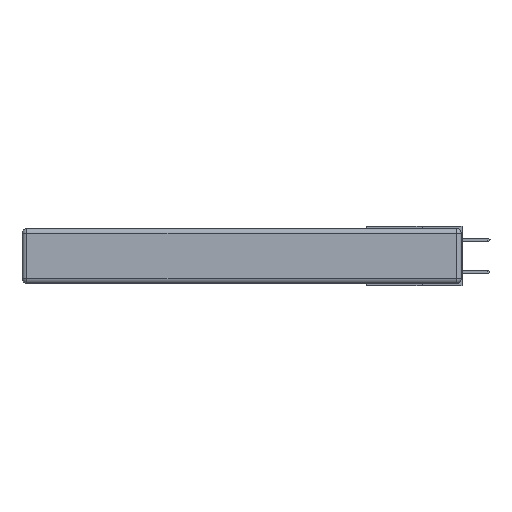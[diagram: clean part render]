
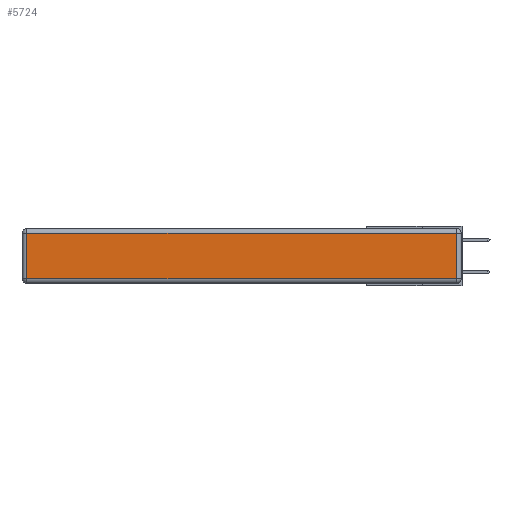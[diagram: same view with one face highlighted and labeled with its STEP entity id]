
A CAD part, left-side view. The second image highlights one B-rep face of the part: STEP entity #5724.
In plain terms, the highlighted planar face has unit normal (-1, 0, 0).
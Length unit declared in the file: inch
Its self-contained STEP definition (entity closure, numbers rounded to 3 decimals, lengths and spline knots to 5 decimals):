
#425 = CARTESIAN_POINT ( 'NONE',  ( 0., 0., -0.343 ) ) ;
#998 = CARTESIAN_POINT ( 'NONE',  ( 0., 2.72, -0.313 ) ) ;
#1907 = EDGE_CURVE ( 'NONE', #13827, #5685, #7964, .T. ) ;
#1959 = VECTOR ( 'NONE', #6742, 39.37008 ) ;
#2517 = DIRECTION ( 'NONE',  ( -1., 0., 0. ) ) ;
#2573 = DIRECTION ( 'NONE',  ( 0., 0., 1. ) ) ;
#3725 = ORIENTED_EDGE ( 'NONE', *, *, #9634, .T. ) ;
#4074 = DIRECTION ( 'NONE',  ( 0., 0., -1. ) ) ;
#4792 = VERTEX_POINT ( 'NONE', #12537 ) ;
#5685 = VERTEX_POINT ( 'NONE', #10365 ) ;
#5724 = ADVANCED_FACE ( 'NONE', ( #11742 ), #8298, .T. ) ;
#5880 = ORIENTED_EDGE ( 'NONE', *, *, #1907, .T. ) ;
#6145 = VECTOR ( 'NONE', #4074, 39.37008 ) ;
#6176 = CARTESIAN_POINT ( 'NONE',  ( 0., 2.75, -0.03 ) ) ;
#6742 = DIRECTION ( 'NONE',  ( 0., 0., 1. ) ) ;
#6750 = ORIENTED_EDGE ( 'NONE', *, *, #9700, .T. ) ;
#6792 = LINE ( 'NONE', #8973, #1959 ) ;
#6838 = DIRECTION ( 'NONE',  ( 0., -1., 0. ) ) ;
#7444 = VECTOR ( 'NONE', #6838, 39.37008 ) ;
#7964 = LINE ( 'NONE', #12325, #7444 ) ;
#8114 = VECTOR ( 'NONE', #8512, 39.37008 ) ;
#8298 = PLANE ( 'NONE',  #14353 ) ;
#8512 = DIRECTION ( 'NONE',  ( 0., 1., 0. ) ) ;
#8834 = CARTESIAN_POINT ( 'NONE',  ( 0., 2.72, -0.03 ) ) ;
#8973 = CARTESIAN_POINT ( 'NONE',  ( 0., 0.03, -0.343 ) ) ;
#9373 = EDGE_LOOP ( 'NONE', ( #5880, #12883, #6750, #3725 ) ) ;
#9512 = LINE ( 'NONE', #6176, #8114 ) ;
#9634 = EDGE_CURVE ( 'NONE', #11934, #13827, #12175, .T. ) ;
#9700 = EDGE_CURVE ( 'NONE', #4792, #11934, #9512, .T. ) ;
#10365 = CARTESIAN_POINT ( 'NONE',  ( 0., 0.03, -0.313 ) ) ;
#11742 = FACE_OUTER_BOUND ( 'NONE', #9373, .T. ) ;
#11934 = VERTEX_POINT ( 'NONE', #8834 ) ;
#11936 = EDGE_CURVE ( 'NONE', #5685, #4792, #6792, .T. ) ;
#12175 = LINE ( 'NONE', #13068, #6145 ) ;
#12325 = CARTESIAN_POINT ( 'NONE',  ( 0., 0., -0.313 ) ) ;
#12537 = CARTESIAN_POINT ( 'NONE',  ( 0., 0.03, -0.03 ) ) ;
#12883 = ORIENTED_EDGE ( 'NONE', *, *, #11936, .T. ) ;
#13068 = CARTESIAN_POINT ( 'NONE',  ( 0., 2.72, -0.343 ) ) ;
#13827 = VERTEX_POINT ( 'NONE', #998 ) ;
#14353 = AXIS2_PLACEMENT_3D ( 'NONE', #425, #2517, #2573 ) ;
